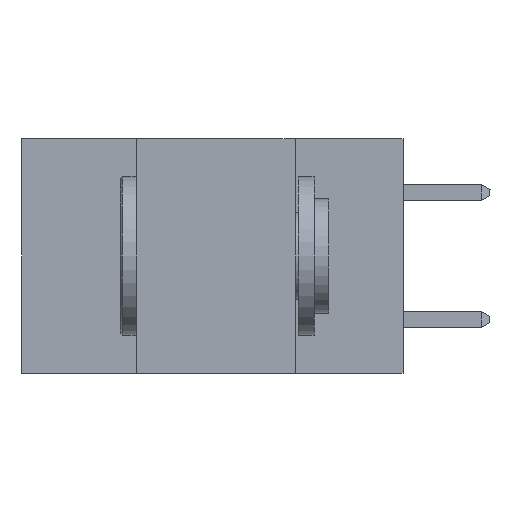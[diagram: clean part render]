
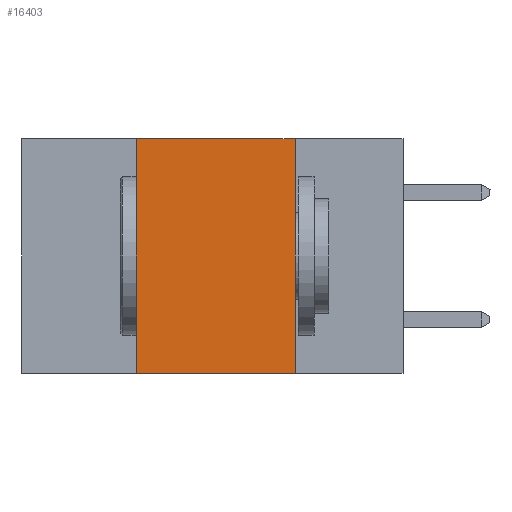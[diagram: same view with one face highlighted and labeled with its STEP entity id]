
A CAD part, left-side view. The second image highlights one B-rep face of the part: STEP entity #16403.
In plain terms, the highlighted planar face has unit normal (-1, 0, 0).
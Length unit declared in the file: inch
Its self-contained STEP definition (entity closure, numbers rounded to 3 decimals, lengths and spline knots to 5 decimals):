
#88 = LINE ( 'NONE', #22797, #23035 ) ;
#1062 = PLANE ( 'NONE',  #8350 ) ;
#5557 = CARTESIAN_POINT ( 'NONE',  ( 0., 0.42, -0.37 ) ) ;
#5958 = CARTESIAN_POINT ( 'NONE',  ( 0., 0.17, 0. ) ) ;
#7078 = DIRECTION ( 'NONE',  ( 0., 0., 1. ) ) ;
#7743 = LINE ( 'NONE', #10289, #16078 ) ;
#7924 = EDGE_CURVE ( 'NONE', #19691, #16129, #7743, .T. ) ;
#8350 = AXIS2_PLACEMENT_3D ( 'NONE', #10307, #10022, #23652 ) ;
#8465 = VECTOR ( 'NONE', #28029, 39.37008 ) ;
#9465 = DIRECTION ( 'NONE',  ( 0., -1., 0. ) ) ;
#10022 = DIRECTION ( 'NONE',  ( 1., 0., 0. ) ) ;
#10289 = CARTESIAN_POINT ( 'NONE',  ( 0., 0.42, 0. ) ) ;
#10307 = CARTESIAN_POINT ( 'NONE',  ( 0., 0.6, 0. ) ) ;
#11883 = EDGE_CURVE ( 'NONE', #19691, #24748, #22536, .T. ) ;
#12701 = ORIENTED_EDGE ( 'NONE', *, *, #22886, .F. ) ;
#14740 = ORIENTED_EDGE ( 'NONE', *, *, #7924, .F. ) ;
#15404 = FACE_OUTER_BOUND ( 'NONE', #26402, .T. ) ;
#15711 = CARTESIAN_POINT ( 'NONE',  ( 0., 0.42, 0. ) ) ;
#16078 = VECTOR ( 'NONE', #7078, 39.37008 ) ;
#16129 = VERTEX_POINT ( 'NONE', #15711 ) ;
#16333 = EDGE_CURVE ( 'NONE', #25163, #24748, #28649, .T. ) ;
#16403 = ADVANCED_FACE ( 'NONE', ( #15404 ), #1062, .F. ) ;
#17648 = CARTESIAN_POINT ( 'NONE',  ( 0., 0.6, -0.37 ) ) ;
#19691 = VERTEX_POINT ( 'NONE', #5557 ) ;
#21595 = ORIENTED_EDGE ( 'NONE', *, *, #16333, .F. ) ;
#22522 = CARTESIAN_POINT ( 'NONE',  ( 0., 0.17, 0. ) ) ;
#22536 = LINE ( 'NONE', #17648, #28130 ) ;
#22797 = CARTESIAN_POINT ( 'NONE',  ( 0., 0.6, 0. ) ) ;
#22886 = EDGE_CURVE ( 'NONE', #16129, #25163, #88, .T. ) ;
#23035 = VECTOR ( 'NONE', #9465, 39.37008 ) ;
#23652 = DIRECTION ( 'NONE',  ( 0., 0., -1. ) ) ;
#24748 = VERTEX_POINT ( 'NONE', #27339 ) ;
#24835 = ORIENTED_EDGE ( 'NONE', *, *, #11883, .T. ) ;
#25163 = VERTEX_POINT ( 'NONE', #5958 ) ;
#26402 = EDGE_LOOP ( 'NONE', ( #21595, #12701, #14740, #24835 ) ) ;
#26708 = DIRECTION ( 'NONE',  ( 0., -1., 0. ) ) ;
#27339 = CARTESIAN_POINT ( 'NONE',  ( 0., 0.17, -0.37 ) ) ;
#28029 = DIRECTION ( 'NONE',  ( 0., 0., -1. ) ) ;
#28130 = VECTOR ( 'NONE', #26708, 39.37008 ) ;
#28649 = LINE ( 'NONE', #22522, #8465 ) ;
